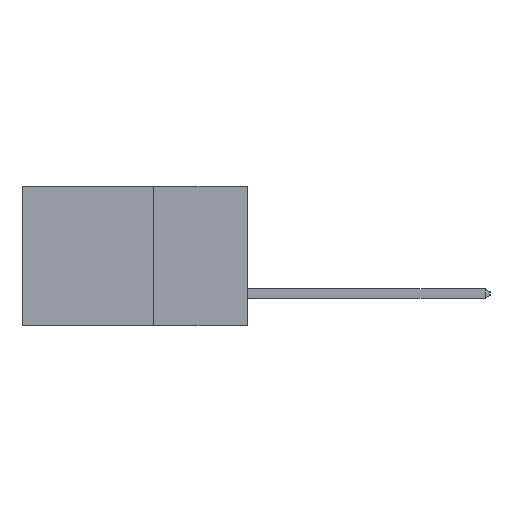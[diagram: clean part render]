
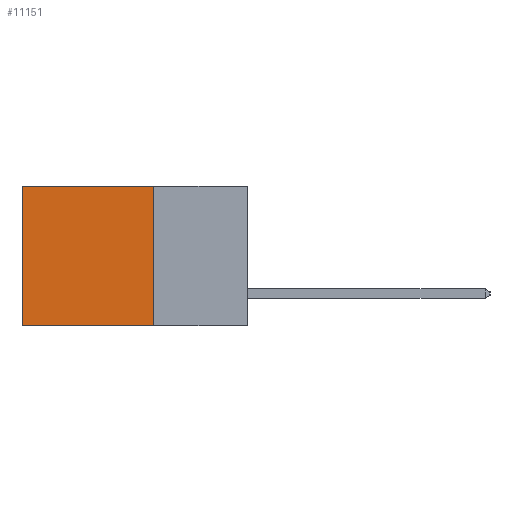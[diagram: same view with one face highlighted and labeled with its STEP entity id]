
A CAD part, left-side view. The second image highlights one B-rep face of the part: STEP entity #11151.
In plain terms, the highlighted planar face has unit normal (-1, 0, 0).
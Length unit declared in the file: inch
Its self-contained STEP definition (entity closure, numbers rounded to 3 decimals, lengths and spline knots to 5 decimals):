
#433 = CARTESIAN_POINT ( 'NONE',  ( 0.298, 0.6, 0. ) ) ;
#877 = EDGE_CURVE ( 'NONE', #1882, #2978, #8924, .T. ) ;
#1299 = VECTOR ( 'NONE', #6291, 39.37008 ) ;
#1882 = VERTEX_POINT ( 'NONE', #5633 ) ;
#2654 = CARTESIAN_POINT ( 'NONE',  ( 0.298, 0.6, 0. ) ) ;
#2862 = DIRECTION ( 'NONE',  ( 1., 0., 0. ) ) ;
#2978 = VERTEX_POINT ( 'NONE', #6766 ) ;
#3391 = LINE ( 'NONE', #2654, #10702 ) ;
#3802 = ORIENTED_EDGE ( 'NONE', *, *, #10166, .T. ) ;
#4130 = ORIENTED_EDGE ( 'NONE', *, *, #877, .F. ) ;
#4316 = CARTESIAN_POINT ( 'NONE',  ( 0.298, 0.25, 0. ) ) ;
#4339 = LINE ( 'NONE', #7989, #6018 ) ;
#4415 = VERTEX_POINT ( 'NONE', #433 ) ;
#4771 = VERTEX_POINT ( 'NONE', #7004 ) ;
#4835 = FACE_OUTER_BOUND ( 'NONE', #8859, .T. ) ;
#5633 = CARTESIAN_POINT ( 'NONE',  ( 0.298, 0.25, 0. ) ) ;
#6018 = VECTOR ( 'NONE', #9732, 39.37008 ) ;
#6195 = VECTOR ( 'NONE', #8908, 39.37008 ) ;
#6291 = DIRECTION ( 'NONE',  ( 0., 0., -1. ) ) ;
#6766 = CARTESIAN_POINT ( 'NONE',  ( 0.298, 0.25, -0.37 ) ) ;
#7004 = CARTESIAN_POINT ( 'NONE',  ( 0.298, 0.6, -0.37 ) ) ;
#7212 = AXIS2_PLACEMENT_3D ( 'NONE', #11985, #2862, #9392 ) ;
#7989 = CARTESIAN_POINT ( 'NONE',  ( 0.298, 0.25, -0.37 ) ) ;
#8355 = DIRECTION ( 'NONE',  ( 0., 0., -1. ) ) ;
#8525 = PLANE ( 'NONE',  #7212 ) ;
#8766 = ORIENTED_EDGE ( 'NONE', *, *, #12216, .F. ) ;
#8859 = EDGE_LOOP ( 'NONE', ( #3802, #8766, #4130, #9034 ) ) ;
#8908 = DIRECTION ( 'NONE',  ( 0., 1., 0. ) ) ;
#8924 = LINE ( 'NONE', #10130, #1299 ) ;
#9034 = ORIENTED_EDGE ( 'NONE', *, *, #10704, .T. ) ;
#9392 = DIRECTION ( 'NONE',  ( 0., 0., -1. ) ) ;
#9732 = DIRECTION ( 'NONE',  ( 0., 1., 0. ) ) ;
#10130 = CARTESIAN_POINT ( 'NONE',  ( 0.298, 0.25, 0. ) ) ;
#10166 = EDGE_CURVE ( 'NONE', #4415, #4771, #3391, .T. ) ;
#10702 = VECTOR ( 'NONE', #8355, 39.37008 ) ;
#10704 = EDGE_CURVE ( 'NONE', #1882, #4415, #11163, .T. ) ;
#11151 = ADVANCED_FACE ( 'NONE', ( #4835 ), #8525, .F. ) ;
#11163 = LINE ( 'NONE', #4316, #6195 ) ;
#11985 = CARTESIAN_POINT ( 'NONE',  ( 0.298, 0.25, 0. ) ) ;
#12216 = EDGE_CURVE ( 'NONE', #2978, #4771, #4339, .T. ) ;
